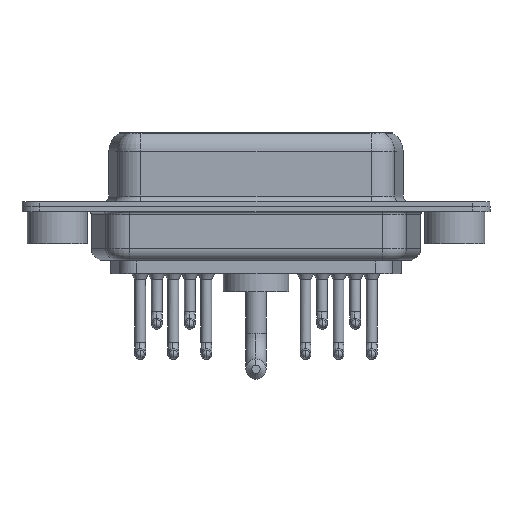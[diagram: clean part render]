
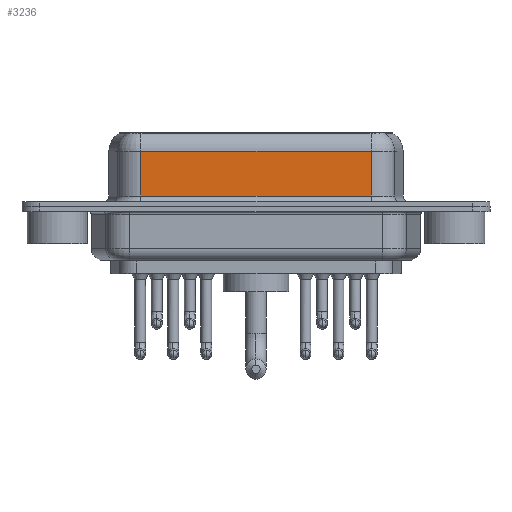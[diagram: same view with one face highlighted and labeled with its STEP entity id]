
A CAD part, front view. The second image highlights one B-rep face of the part: STEP entity #3236.
In plain terms, the highlighted planar face has unit normal (0, -1, 0).
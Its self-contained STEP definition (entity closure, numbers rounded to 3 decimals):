
#716 = LINE ( 'NONE', #5194, #1758 ) ;
#889 = FACE_OUTER_BOUND ( 'NONE', #7370, .T. ) ;
#1144 = VECTOR ( 'NONE', #17556, 1000. ) ;
#1656 = EDGE_CURVE ( 'NONE', #16417, #11853, #716, .T. ) ;
#1758 = VECTOR ( 'NONE', #10940, 1000. ) ;
#2666 = CARTESIAN_POINT ( 'NONE',  ( 7.013, -3.95, 4.65 ) ) ;
#3236 = ADVANCED_FACE ( 'NONE', ( #889 ), #6491, .F. ) ;
#4340 = LINE ( 'NONE', #17566, #8954 ) ;
#4720 = DIRECTION ( 'NONE',  ( 0., 0., -1. ) ) ;
#4990 = CARTESIAN_POINT ( 'NONE',  ( 26.287, -3.95, 6.4 ) ) ;
#5194 = CARTESIAN_POINT ( 'NONE',  ( 7.013, -3.95, 6.4 ) ) ;
#5490 = CARTESIAN_POINT ( 'NONE',  ( 7.013, -3.95, 0.9 ) ) ;
#6129 = ORIENTED_EDGE ( 'NONE', *, *, #12204, .T. ) ;
#6153 = LINE ( 'NONE', #11621, #16400 ) ;
#6491 = PLANE ( 'NONE',  #16466 ) ;
#6674 = DIRECTION ( 'NONE',  ( 0., 1., 0. ) ) ;
#7345 = LINE ( 'NONE', #17457, #1144 ) ;
#7370 = EDGE_LOOP ( 'NONE', ( #10432, #6129, #16227, #17948 ) ) ;
#7840 = EDGE_CURVE ( 'NONE', #13818, #15177, #4340, .T. ) ;
#8954 = VECTOR ( 'NONE', #4720, 1000. ) ;
#9487 = CARTESIAN_POINT ( 'NONE',  ( 26.287, -3.95, 4.65 ) ) ;
#10432 = ORIENTED_EDGE ( 'NONE', *, *, #7840, .F. ) ;
#10609 = EDGE_CURVE ( 'NONE', #11853, #15177, #6153, .T. ) ;
#10940 = DIRECTION ( 'NONE',  ( 0., 0., -1. ) ) ;
#11621 = CARTESIAN_POINT ( 'NONE',  ( 26.287, -3.95, 0.9 ) ) ;
#11853 = VERTEX_POINT ( 'NONE', #5490 ) ;
#12204 = EDGE_CURVE ( 'NONE', #13818, #16417, #7345, .T. ) ;
#13677 = DIRECTION ( 'NONE',  ( 0., 0., 1. ) ) ;
#13818 = VERTEX_POINT ( 'NONE', #9487 ) ;
#15177 = VERTEX_POINT ( 'NONE', #15207 ) ;
#15207 = CARTESIAN_POINT ( 'NONE',  ( 26.287, -3.95, 0.9 ) ) ;
#16227 = ORIENTED_EDGE ( 'NONE', *, *, #1656, .T. ) ;
#16400 = VECTOR ( 'NONE', #17486, 1000. ) ;
#16417 = VERTEX_POINT ( 'NONE', #2666 ) ;
#16466 = AXIS2_PLACEMENT_3D ( 'NONE', #4990, #6674, #13677 ) ;
#17457 = CARTESIAN_POINT ( 'NONE',  ( 26.287, -3.95, 4.65 ) ) ;
#17486 = DIRECTION ( 'NONE',  ( 1., 0., 0. ) ) ;
#17556 = DIRECTION ( 'NONE',  ( -1., 0., 0. ) ) ;
#17566 = CARTESIAN_POINT ( 'NONE',  ( 26.287, -3.95, 6.4 ) ) ;
#17948 = ORIENTED_EDGE ( 'NONE', *, *, #10609, .T. ) ;
